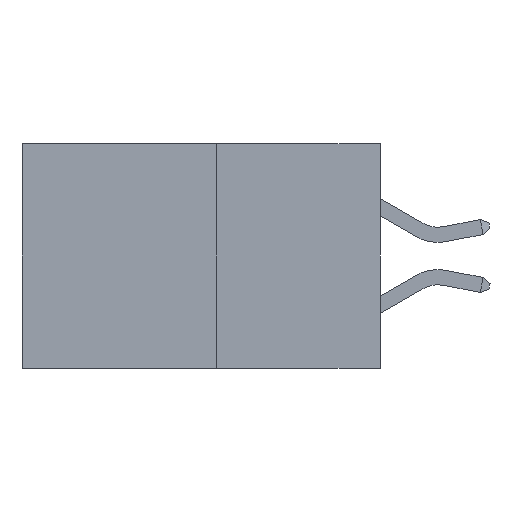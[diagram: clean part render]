
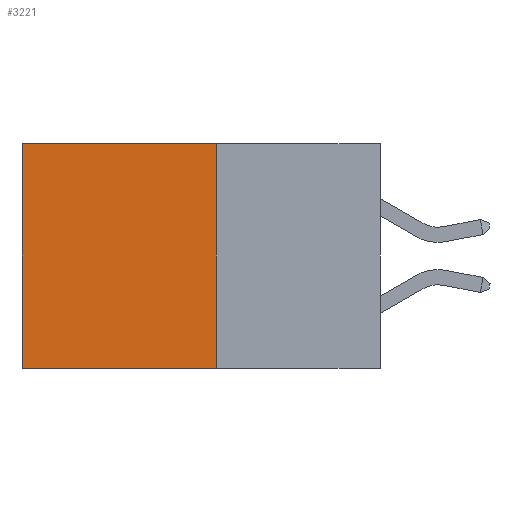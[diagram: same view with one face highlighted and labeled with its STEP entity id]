
A CAD part, left-side view. The second image highlights one B-rep face of the part: STEP entity #3221.
In plain terms, the highlighted planar face has unit normal (-1, 0, 0).
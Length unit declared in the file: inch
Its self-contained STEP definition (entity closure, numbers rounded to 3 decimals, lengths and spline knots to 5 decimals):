
#84 = CARTESIAN_POINT ( 'NONE',  ( 0.277, 0.59, 0. ) ) ;
#129 = CARTESIAN_POINT ( 'NONE',  ( 0.277, 0.27, -0.37 ) ) ;
#722 = ORIENTED_EDGE ( 'NONE', *, *, #5673, .F. ) ;
#1064 = VECTOR ( 'NONE', #1823, 39.37008 ) ;
#1185 = CARTESIAN_POINT ( 'NONE',  ( 0.277, 0.59, -0.37 ) ) ;
#1823 = DIRECTION ( 'NONE',  ( 0., 0., -1. ) ) ;
#1916 = FACE_OUTER_BOUND ( 'NONE', #5052, .T. ) ;
#2302 = CARTESIAN_POINT ( 'NONE',  ( 0.277, 0.59, -0.37 ) ) ;
#2427 = VERTEX_POINT ( 'NONE', #2899 ) ;
#2431 = DIRECTION ( 'NONE',  ( 0., 1., 0. ) ) ;
#2641 = ORIENTED_EDGE ( 'NONE', *, *, #5413, .F. ) ;
#2899 = CARTESIAN_POINT ( 'NONE',  ( 0.277, 0.27, 0. ) ) ;
#3059 = CARTESIAN_POINT ( 'NONE',  ( 0.277, 0.27, 0. ) ) ;
#3115 = PLANE ( 'NONE',  #3247 ) ;
#3221 = ADVANCED_FACE ( 'NONE', ( #1916 ), #3115, .F. ) ;
#3247 = AXIS2_PLACEMENT_3D ( 'NONE', #129, #7248, #7269 ) ;
#3396 = VERTEX_POINT ( 'NONE', #2302 ) ;
#3463 = EDGE_CURVE ( 'NONE', #2427, #6042, #7104, .T. ) ;
#3847 = EDGE_CURVE ( 'NONE', #6042, #3396, #4855, .T. ) ;
#4068 = VECTOR ( 'NONE', #2431, 39.37008 ) ;
#4259 = LINE ( 'NONE', #7638, #4068 ) ;
#4641 = CARTESIAN_POINT ( 'NONE',  ( 0.277, 0.27, -0.37 ) ) ;
#4855 = LINE ( 'NONE', #1185, #1064 ) ;
#5052 = EDGE_LOOP ( 'NONE', ( #7298, #722, #2641, #6020 ) ) ;
#5202 = CARTESIAN_POINT ( 'NONE',  ( 0.277, 0.27, -0.37 ) ) ;
#5413 = EDGE_CURVE ( 'NONE', #2427, #6433, #6490, .T. ) ;
#5673 = EDGE_CURVE ( 'NONE', #6433, #3396, #4259, .T. ) ;
#6020 = ORIENTED_EDGE ( 'NONE', *, *, #3463, .T. ) ;
#6042 = VERTEX_POINT ( 'NONE', #84 ) ;
#6292 = VECTOR ( 'NONE', #7094, 39.37008 ) ;
#6433 = VERTEX_POINT ( 'NONE', #5202 ) ;
#6490 = LINE ( 'NONE', #4641, #6292 ) ;
#6957 = VECTOR ( 'NONE', #7232, 39.37008 ) ;
#7094 = DIRECTION ( 'NONE',  ( 0., 0., -1. ) ) ;
#7104 = LINE ( 'NONE', #3059, #6957 ) ;
#7232 = DIRECTION ( 'NONE',  ( 0., 1., 0. ) ) ;
#7248 = DIRECTION ( 'NONE',  ( 1., 0., 0. ) ) ;
#7269 = DIRECTION ( 'NONE',  ( 0., 0., -1. ) ) ;
#7298 = ORIENTED_EDGE ( 'NONE', *, *, #3847, .T. ) ;
#7638 = CARTESIAN_POINT ( 'NONE',  ( 0.277, 0.27, -0.37 ) ) ;
